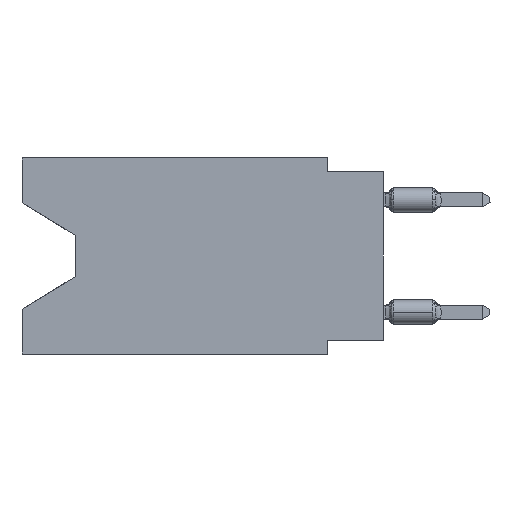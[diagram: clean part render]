
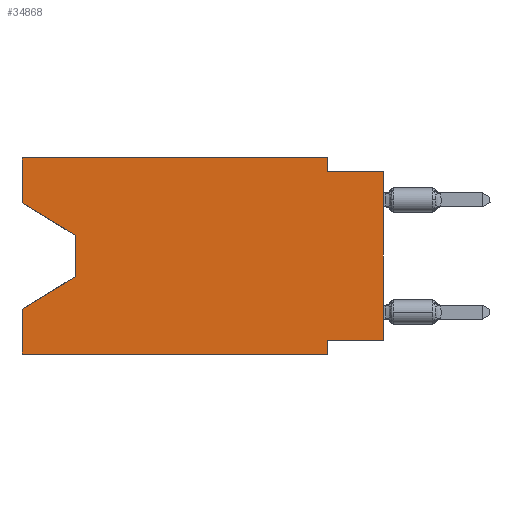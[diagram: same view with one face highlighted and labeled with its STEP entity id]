
A CAD part, left-side view. The second image highlights one B-rep face of the part: STEP entity #34868.
In plain terms, the highlighted planar face has unit normal (-1, 0, 0).
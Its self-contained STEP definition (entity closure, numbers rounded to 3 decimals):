
#273 = EDGE_CURVE ( 'NONE', #24589, #26280, #19272, .T. ) ;
#1685 = LINE ( 'NONE', #2221, #43547 ) ;
#1753 = DIRECTION ( 'NONE',  ( 0., -1., 0. ) ) ;
#1925 = CARTESIAN_POINT ( 'NONE',  ( 0., 16.383, 0. ) ) ;
#2064 = EDGE_CURVE ( 'NONE', #30522, #15625, #10298, .T. ) ;
#2144 = VECTOR ( 'NONE', #37466, 1000. ) ;
#2221 = CARTESIAN_POINT ( 'NONE',  ( 0., 13.97, -5.385 ) ) ;
#2401 = ORIENTED_EDGE ( 'NONE', *, *, #47096, .T. ) ;
#2791 = LINE ( 'NONE', #5690, #9166 ) ;
#2980 = DIRECTION ( 'NONE',  ( 0., 0., -1. ) ) ;
#4753 = AXIS2_PLACEMENT_3D ( 'NONE', #37400, #30310, #26376 ) ;
#4777 = ORIENTED_EDGE ( 'NONE', *, *, #39341, .F. ) ;
#5020 = VERTEX_POINT ( 'NONE', #50957 ) ;
#5095 = EDGE_CURVE ( 'NONE', #43092, #23529, #40674, .T. ) ;
#5441 = LINE ( 'NONE', #21459, #2144 ) ;
#5690 = CARTESIAN_POINT ( 'NONE',  ( 0., 16.383, -8.89 ) ) ;
#5732 = LINE ( 'NONE', #26464, #28825 ) ;
#5780 = LINE ( 'NONE', #45418, #30272 ) ;
#6576 = ORIENTED_EDGE ( 'NONE', *, *, #49946, .F. ) ;
#7692 = CARTESIAN_POINT ( 'NONE',  ( 0., 13.97, -3.505 ) ) ;
#8687 = VECTOR ( 'NONE', #44763, 1000. ) ;
#9166 = VECTOR ( 'NONE', #1753, 1000. ) ;
#10049 = CARTESIAN_POINT ( 'NONE',  ( 0., 13.97, -3.505 ) ) ;
#10298 = LINE ( 'NONE', #22377, #29419 ) ;
#11752 = EDGE_CURVE ( 'NONE', #26466, #46397, #39456, .T. ) ;
#13018 = LINE ( 'NONE', #17723, #8687 ) ;
#14293 = FACE_OUTER_BOUND ( 'NONE', #20948, .T. ) ;
#15184 = CARTESIAN_POINT ( 'NONE',  ( 0., 13.97, -5.385 ) ) ;
#15625 = VERTEX_POINT ( 'NONE', #23500 ) ;
#16285 = CARTESIAN_POINT ( 'NONE',  ( 0., 16.383, 0. ) ) ;
#17723 = CARTESIAN_POINT ( 'NONE',  ( 0., 16.383, -2.038 ) ) ;
#17857 = EDGE_CURVE ( 'NONE', #23529, #30522, #5732, .T. ) ;
#17983 = CARTESIAN_POINT ( 'NONE',  ( 0., 0., -0.635 ) ) ;
#19272 = LINE ( 'NONE', #23722, #37659 ) ;
#20948 = EDGE_LOOP ( 'NONE', ( #47908, #28871, #2401, #36323, #34688, #6576, #28987, #48761, #4777, #39450, #26964, #32061 ) ) ;
#21459 = CARTESIAN_POINT ( 'NONE',  ( 0., 0., 0. ) ) ;
#22182 = LINE ( 'NONE', #17983, #50689 ) ;
#22377 = CARTESIAN_POINT ( 'NONE',  ( 0., 2.54, 0. ) ) ;
#22520 = CARTESIAN_POINT ( 'NONE',  ( 0., 16.383, 0. ) ) ;
#23500 = CARTESIAN_POINT ( 'NONE',  ( 0., 2.54, -0.635 ) ) ;
#23529 = VERTEX_POINT ( 'NONE', #22520 ) ;
#23722 = CARTESIAN_POINT ( 'NONE',  ( 0., 0., -8.255 ) ) ;
#24419 = DIRECTION ( 'NONE',  ( 0., 0., 1. ) ) ;
#24589 = VERTEX_POINT ( 'NONE', #33209 ) ;
#24610 = EDGE_CURVE ( 'NONE', #43092, #26466, #13018, .T. ) ;
#26181 = EDGE_CURVE ( 'NONE', #36116, #42364, #40772, .T. ) ;
#26280 = VERTEX_POINT ( 'NONE', #29744 ) ;
#26317 = DIRECTION ( 'NONE',  ( 0., 0., -1. ) ) ;
#26376 = DIRECTION ( 'NONE',  ( 0., 0., -1. ) ) ;
#26464 = CARTESIAN_POINT ( 'NONE',  ( 0., 16.383, 0. ) ) ;
#26466 = VERTEX_POINT ( 'NONE', #10049 ) ;
#26964 = ORIENTED_EDGE ( 'NONE', *, *, #17857, .F. ) ;
#27146 = DIRECTION ( 'NONE',  ( 0., 1., 0. ) ) ;
#28825 = VECTOR ( 'NONE', #29886, 1000. ) ;
#28871 = ORIENTED_EDGE ( 'NONE', *, *, #11752, .T. ) ;
#28987 = ORIENTED_EDGE ( 'NONE', *, *, #273, .F. ) ;
#29419 = VECTOR ( 'NONE', #26317, 1000. ) ;
#29744 = CARTESIAN_POINT ( 'NONE',  ( 0., 2.54, -8.255 ) ) ;
#29886 = DIRECTION ( 'NONE',  ( 0., -1., 0. ) ) ;
#30064 = DIRECTION ( 'NONE',  ( 0., -1., 0. ) ) ;
#30272 = VECTOR ( 'NONE', #49617, 1000. ) ;
#30310 = DIRECTION ( 'NONE',  ( 1., 0., 0. ) ) ;
#30498 = CARTESIAN_POINT ( 'NONE',  ( 0., 0., -0.635 ) ) ;
#30522 = VERTEX_POINT ( 'NONE', #50061 ) ;
#32061 = ORIENTED_EDGE ( 'NONE', *, *, #5095, .F. ) ;
#33209 = CARTESIAN_POINT ( 'NONE',  ( 0., 0., -8.255 ) ) ;
#33294 = EDGE_CURVE ( 'NONE', #24589, #36849, #5441, .T. ) ;
#34688 = ORIENTED_EDGE ( 'NONE', *, *, #46798, .T. ) ;
#34868 = ADVANCED_FACE ( 'NONE', ( #14293 ), #46047, .F. ) ;
#36116 = VERTEX_POINT ( 'NONE', #45398 ) ;
#36323 = ORIENTED_EDGE ( 'NONE', *, *, #26181, .F. ) ;
#36849 = VERTEX_POINT ( 'NONE', #30498 ) ;
#37400 = CARTESIAN_POINT ( 'NONE',  ( 0., 16.383, 0. ) ) ;
#37466 = DIRECTION ( 'NONE',  ( 0., 0., 1. ) ) ;
#37659 = VECTOR ( 'NONE', #27146, 1000. ) ;
#38801 = CARTESIAN_POINT ( 'NONE',  ( 0., 16.383, -2.038 ) ) ;
#39341 = EDGE_CURVE ( 'NONE', #15625, #36849, #22182, .T. ) ;
#39450 = ORIENTED_EDGE ( 'NONE', *, *, #2064, .F. ) ;
#39456 = LINE ( 'NONE', #7692, #40883 ) ;
#40674 = LINE ( 'NONE', #16285, #49646 ) ;
#40772 = LINE ( 'NONE', #1925, #49906 ) ;
#40883 = VECTOR ( 'NONE', #2980, 1000. ) ;
#42364 = VERTEX_POINT ( 'NONE', #44648 ) ;
#43092 = VERTEX_POINT ( 'NONE', #38801 ) ;
#43547 = VECTOR ( 'NONE', #50498, 1000. ) ;
#44648 = CARTESIAN_POINT ( 'NONE',  ( 0., 16.383, -6.852 ) ) ;
#44763 = DIRECTION ( 'NONE',  ( 0., -0.855, -0.519 ) ) ;
#45398 = CARTESIAN_POINT ( 'NONE',  ( 0., 16.383, -8.89 ) ) ;
#45418 = CARTESIAN_POINT ( 'NONE',  ( 0., 2.54, -8.89 ) ) ;
#46047 = PLANE ( 'NONE',  #4753 ) ;
#46397 = VERTEX_POINT ( 'NONE', #15184 ) ;
#46798 = EDGE_CURVE ( 'NONE', #36116, #5020, #2791, .T. ) ;
#47096 = EDGE_CURVE ( 'NONE', #46397, #42364, #1685, .T. ) ;
#47908 = ORIENTED_EDGE ( 'NONE', *, *, #24610, .T. ) ;
#48761 = ORIENTED_EDGE ( 'NONE', *, *, #33294, .T. ) ;
#49617 = DIRECTION ( 'NONE',  ( 0., 0., -1. ) ) ;
#49646 = VECTOR ( 'NONE', #24419, 1000. ) ;
#49688 = DIRECTION ( 'NONE',  ( 0., 0., 1. ) ) ;
#49906 = VECTOR ( 'NONE', #49688, 1000. ) ;
#49946 = EDGE_CURVE ( 'NONE', #26280, #5020, #5780, .T. ) ;
#50061 = CARTESIAN_POINT ( 'NONE',  ( 0., 2.54, 0. ) ) ;
#50498 = DIRECTION ( 'NONE',  ( 0., 0.855, -0.519 ) ) ;
#50689 = VECTOR ( 'NONE', #30064, 1000. ) ;
#50957 = CARTESIAN_POINT ( 'NONE',  ( 0., 2.54, -8.89 ) ) ;
